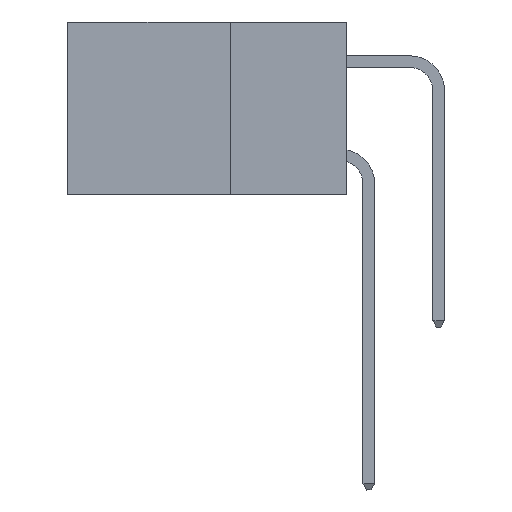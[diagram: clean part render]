
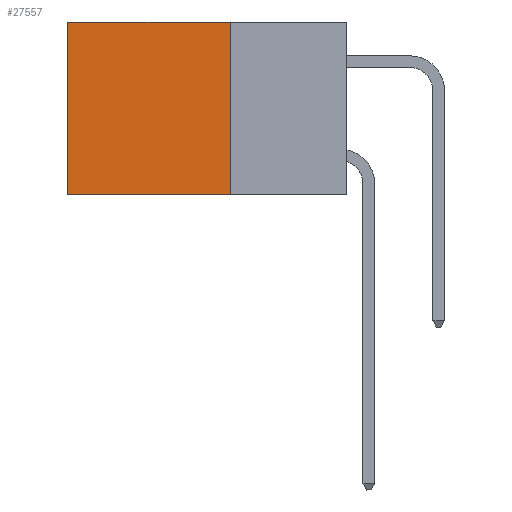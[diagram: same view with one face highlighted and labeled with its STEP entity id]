
A CAD part, left-side view. The second image highlights one B-rep face of the part: STEP entity #27557.
In plain terms, the highlighted planar face has unit normal (-1, 0, 0).
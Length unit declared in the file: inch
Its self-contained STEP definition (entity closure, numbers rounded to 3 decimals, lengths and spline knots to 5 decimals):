
#1120 = VERTEX_POINT ( 'NONE', #23004 ) ;
#1435 = CARTESIAN_POINT ( 'NONE',  ( 0.2875, 0.25, 0. ) ) ;
#3975 = VECTOR ( 'NONE', #5750, 39.37008 ) ;
#5386 = VERTEX_POINT ( 'NONE', #34116 ) ;
#5750 = DIRECTION ( 'NONE',  ( 0., 1., 0. ) ) ;
#6594 = CARTESIAN_POINT ( 'NONE',  ( 0.2875, 0.6, 0. ) ) ;
#7377 = ORIENTED_EDGE ( 'NONE', *, *, #33711, .T. ) ;
#8754 = EDGE_CURVE ( 'NONE', #5386, #16523, #17856, .T. ) ;
#11526 = ORIENTED_EDGE ( 'NONE', *, *, #24013, .F. ) ;
#13243 = VECTOR ( 'NONE', #25507, 39.37008 ) ;
#13269 = DIRECTION ( 'NONE',  ( 1., 0., 0. ) ) ;
#13767 = LINE ( 'NONE', #24525, #3975 ) ;
#14684 = CARTESIAN_POINT ( 'NONE',  ( 0.2875, 0.25, 0. ) ) ;
#16523 = VERTEX_POINT ( 'NONE', #39230 ) ;
#17484 = EDGE_LOOP ( 'NONE', ( #7377, #11526, #35649, #26018 ) ) ;
#17856 = LINE ( 'NONE', #1435, #32603 ) ;
#20135 = LINE ( 'NONE', #6594, #13243 ) ;
#21827 = FACE_OUTER_BOUND ( 'NONE', #17484, .T. ) ;
#22874 = DIRECTION ( 'NONE',  ( 0., 0., -1. ) ) ;
#23004 = CARTESIAN_POINT ( 'NONE',  ( 0.2875, 0.25, -0.37 ) ) ;
#23416 = EDGE_CURVE ( 'NONE', #5386, #1120, #32449, .T. ) ;
#24013 = EDGE_CURVE ( 'NONE', #1120, #32639, #13767, .T. ) ;
#24525 = CARTESIAN_POINT ( 'NONE',  ( 0.2875, 0.25, -0.37 ) ) ;
#25507 = DIRECTION ( 'NONE',  ( 0., 0., -1. ) ) ;
#26018 = ORIENTED_EDGE ( 'NONE', *, *, #8754, .T. ) ;
#27431 = DIRECTION ( 'NONE',  ( 0., 0., -1. ) ) ;
#27520 = VECTOR ( 'NONE', #27431, 39.37008 ) ;
#27557 = ADVANCED_FACE ( 'NONE', ( #21827 ), #28745, .F. ) ;
#28690 = AXIS2_PLACEMENT_3D ( 'NONE', #31910, #13269, #22874 ) ;
#28745 = PLANE ( 'NONE',  #28690 ) ;
#31910 = CARTESIAN_POINT ( 'NONE',  ( 0.2875, 0.25, 0. ) ) ;
#32449 = LINE ( 'NONE', #14684, #27520 ) ;
#32603 = VECTOR ( 'NONE', #35337, 39.37008 ) ;
#32639 = VERTEX_POINT ( 'NONE', #33830 ) ;
#33711 = EDGE_CURVE ( 'NONE', #16523, #32639, #20135, .T. ) ;
#33830 = CARTESIAN_POINT ( 'NONE',  ( 0.2875, 0.6, -0.37 ) ) ;
#34116 = CARTESIAN_POINT ( 'NONE',  ( 0.2875, 0.25, 0. ) ) ;
#35337 = DIRECTION ( 'NONE',  ( 0., 1., 0. ) ) ;
#35649 = ORIENTED_EDGE ( 'NONE', *, *, #23416, .F. ) ;
#39230 = CARTESIAN_POINT ( 'NONE',  ( 0.2875, 0.6, 0. ) ) ;
